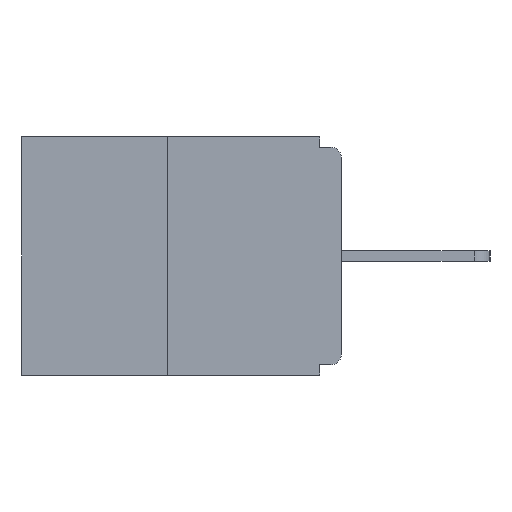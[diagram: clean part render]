
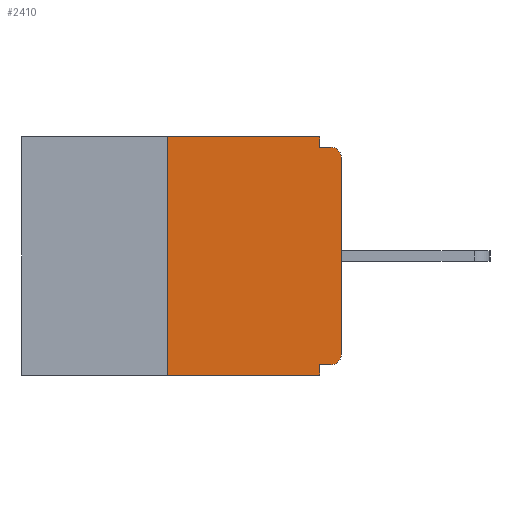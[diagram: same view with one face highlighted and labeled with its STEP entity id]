
A CAD part, left-side view. The second image highlights one B-rep face of the part: STEP entity #2410.
In plain terms, the highlighted planar face has unit normal (-1, 0, 0).
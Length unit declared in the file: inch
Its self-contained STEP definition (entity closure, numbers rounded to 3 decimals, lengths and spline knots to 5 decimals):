
#83 = EDGE_CURVE ( 'NONE', #1155, #16157, #16680, .T. ) ;
#577 = VERTEX_POINT ( 'NONE', #2446 ) ;
#580 = VERTEX_POINT ( 'NONE', #9753 ) ;
#1004 = CARTESIAN_POINT ( 'NONE',  ( 0., 0.031, -0.328 ) ) ;
#1065 = DIRECTION ( 'NONE',  ( 0., 0., -1. ) ) ;
#1155 = VERTEX_POINT ( 'NONE', #14059 ) ;
#2410 = ADVANCED_FACE ( 'NONE', ( #7007 ), #14104, .F. ) ;
#2446 = CARTESIAN_POINT ( 'NONE',  ( 0., 0.031, -0.343 ) ) ;
#2525 = LINE ( 'NONE', #20049, #4802 ) ;
#2542 = CARTESIAN_POINT ( 'NONE',  ( 0., 0.25, 0. ) ) ;
#2829 = ORIENTED_EDGE ( 'NONE', *, *, #18890, .F. ) ;
#3570 = VERTEX_POINT ( 'NONE', #10436 ) ;
#3967 = CARTESIAN_POINT ( 'NONE',  ( 0., 0.031, -0.343 ) ) ;
#4155 = CARTESIAN_POINT ( 'NONE',  ( 0., 0., -0.328 ) ) ;
#4443 = VECTOR ( 'NONE', #13846, 39.37008 ) ;
#4802 = VECTOR ( 'NONE', #9508, 39.37008 ) ;
#4964 = ORIENTED_EDGE ( 'NONE', *, *, #8487, .F. ) ;
#5262 = CARTESIAN_POINT ( 'NONE',  ( 0., 0.46, -0.343 ) ) ;
#5610 = EDGE_CURVE ( 'NONE', #580, #16157, #6360, .T. ) ;
#5783 = DIRECTION ( 'NONE',  ( 0., 1., 0. ) ) ;
#5798 = EDGE_CURVE ( 'NONE', #19102, #21893, #15682, .T. ) ;
#5938 = LINE ( 'NONE', #3967, #15348 ) ;
#5979 = ORIENTED_EDGE ( 'NONE', *, *, #22280, .F. ) ;
#6029 = VECTOR ( 'NONE', #11950, 39.37008 ) ;
#6326 = DIRECTION ( 'NONE',  ( 0., 0., 1. ) ) ;
#6360 = LINE ( 'NONE', #13560, #6029 ) ;
#6496 = CARTESIAN_POINT ( 'NONE',  ( 0., 0.25, -0.343 ) ) ;
#6692 = DIRECTION ( 'NONE',  ( 0., -1., 0. ) ) ;
#7007 = FACE_OUTER_BOUND ( 'NONE', #7883, .T. ) ;
#7710 = LINE ( 'NONE', #4155, #20511 ) ;
#7823 = LINE ( 'NONE', #2542, #16462 ) ;
#7883 = EDGE_LOOP ( 'NONE', ( #5979, #10513, #22159, #4964, #2829, #19132, #9240, #10313, #12474, #9782 ) ) ;
#8487 = EDGE_CURVE ( 'NONE', #9374, #577, #5938, .T. ) ;
#8532 = LINE ( 'NONE', #13793, #19493 ) ;
#8824 = LINE ( 'NONE', #15685, #4443 ) ;
#9240 = ORIENTED_EDGE ( 'NONE', *, *, #21171, .T. ) ;
#9374 = VERTEX_POINT ( 'NONE', #1004 ) ;
#9508 = DIRECTION ( 'NONE',  ( 0., 0., 1. ) ) ;
#9737 = EDGE_CURVE ( 'NONE', #12528, #577, #10515, .T. ) ;
#9753 = CARTESIAN_POINT ( 'NONE',  ( 0., 0.031, -0.015 ) ) ;
#9782 = ORIENTED_EDGE ( 'NONE', *, *, #20745, .F. ) ;
#10188 = EDGE_CURVE ( 'NONE', #12528, #3570, #7823, .T. ) ;
#10219 = CARTESIAN_POINT ( 'NONE',  ( 0., 0.031, 0. ) ) ;
#10313 = ORIENTED_EDGE ( 'NONE', *, *, #83, .T. ) ;
#10436 = CARTESIAN_POINT ( 'NONE',  ( 0., 0.25, 0. ) ) ;
#10450 = AXIS2_PLACEMENT_3D ( 'NONE', #10779, #10658, #17851 ) ;
#10513 = ORIENTED_EDGE ( 'NONE', *, *, #10188, .F. ) ;
#10515 = LINE ( 'NONE', #5262, #20469 ) ;
#10658 = DIRECTION ( 'NONE',  ( 1., 0., 0. ) ) ;
#10779 = CARTESIAN_POINT ( 'NONE',  ( 0., 0.46, 0. ) ) ;
#11950 = DIRECTION ( 'NONE',  ( 0., -1., 0. ) ) ;
#12105 = CARTESIAN_POINT ( 'NONE',  ( 0., 0., -0.313 ) ) ;
#12474 = ORIENTED_EDGE ( 'NONE', *, *, #5610, .F. ) ;
#12528 = VERTEX_POINT ( 'NONE', #6496 ) ;
#13008 = DIRECTION ( 'NONE',  ( -1., 0., 0. ) ) ;
#13560 = CARTESIAN_POINT ( 'NONE',  ( 0., 0., -0.015 ) ) ;
#13793 = CARTESIAN_POINT ( 'NONE',  ( 0., 0.46, 0. ) ) ;
#13846 = DIRECTION ( 'NONE',  ( 0., 0., -1. ) ) ;
#14059 = CARTESIAN_POINT ( 'NONE',  ( 0., 0., -0.03 ) ) ;
#14104 = PLANE ( 'NONE',  #10450 ) ;
#15348 = VECTOR ( 'NONE', #17932, 39.37008 ) ;
#15623 = CARTESIAN_POINT ( 'NONE',  ( 0., 0.015, -0.313 ) ) ;
#15682 = CIRCLE ( 'NONE', #20422, 0.015 ) ;
#15685 = CARTESIAN_POINT ( 'NONE',  ( 0., 0.031, 0. ) ) ;
#15826 = VERTEX_POINT ( 'NONE', #10219 ) ;
#15979 = DIRECTION ( 'NONE',  ( 0., 0., -1. ) ) ;
#16157 = VERTEX_POINT ( 'NONE', #21911 ) ;
#16462 = VECTOR ( 'NONE', #6326, 39.37008 ) ;
#16680 = CIRCLE ( 'NONE', #18155, 0.015 ) ;
#17374 = DIRECTION ( 'NONE',  ( 0., -1., 0. ) ) ;
#17851 = DIRECTION ( 'NONE',  ( 0., 0., -1. ) ) ;
#17932 = DIRECTION ( 'NONE',  ( 0., 0., -1. ) ) ;
#18155 = AXIS2_PLACEMENT_3D ( 'NONE', #18584, #13008, #1065 ) ;
#18584 = CARTESIAN_POINT ( 'NONE',  ( 0., 0.015, -0.03 ) ) ;
#18890 = EDGE_CURVE ( 'NONE', #19102, #9374, #7710, .T. ) ;
#19102 = VERTEX_POINT ( 'NONE', #21915 ) ;
#19132 = ORIENTED_EDGE ( 'NONE', *, *, #5798, .T. ) ;
#19493 = VECTOR ( 'NONE', #6692, 39.37008 ) ;
#20049 = CARTESIAN_POINT ( 'NONE',  ( 0., 0., 0. ) ) ;
#20422 = AXIS2_PLACEMENT_3D ( 'NONE', #15623, #21263, #15979 ) ;
#20469 = VECTOR ( 'NONE', #17374, 39.37008 ) ;
#20511 = VECTOR ( 'NONE', #5783, 39.37008 ) ;
#20745 = EDGE_CURVE ( 'NONE', #15826, #580, #8824, .T. ) ;
#21171 = EDGE_CURVE ( 'NONE', #21893, #1155, #2525, .T. ) ;
#21263 = DIRECTION ( 'NONE',  ( -1., 0., 0. ) ) ;
#21893 = VERTEX_POINT ( 'NONE', #12105 ) ;
#21911 = CARTESIAN_POINT ( 'NONE',  ( 0., 0.015, -0.015 ) ) ;
#21915 = CARTESIAN_POINT ( 'NONE',  ( 0., 0.015, -0.328 ) ) ;
#22159 = ORIENTED_EDGE ( 'NONE', *, *, #9737, .T. ) ;
#22280 = EDGE_CURVE ( 'NONE', #3570, #15826, #8532, .T. ) ;
